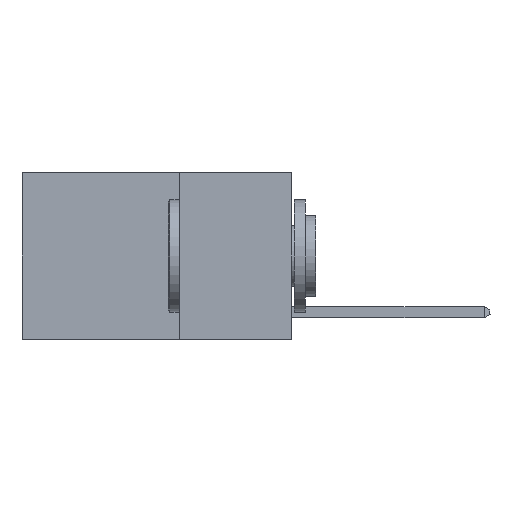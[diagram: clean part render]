
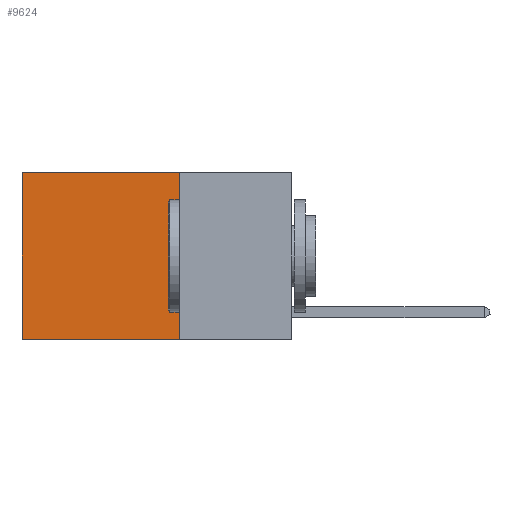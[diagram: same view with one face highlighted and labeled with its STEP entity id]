
A CAD part, left-side view. The second image highlights one B-rep face of the part: STEP entity #9624.
In plain terms, the highlighted planar face has unit normal (-1, 0, 0).
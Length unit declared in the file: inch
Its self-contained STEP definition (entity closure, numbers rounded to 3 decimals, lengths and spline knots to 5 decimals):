
#77 = AXIS2_PLACEMENT_3D ( 'NONE', #5192, #1181, #6206 ) ;
#210 = ORIENTED_EDGE ( 'NONE', *, *, #11978, .F. ) ;
#230 = CARTESIAN_POINT ( 'NONE',  ( 0.2625, 0.6, 0. ) ) ;
#851 = CARTESIAN_POINT ( 'NONE',  ( 0.2625, 0.25, 0. ) ) ;
#937 = DIRECTION ( 'NONE',  ( 0., 0., -1. ) ) ;
#1181 = DIRECTION ( 'NONE',  ( 1., 0., 0. ) ) ;
#1948 = CARTESIAN_POINT ( 'NONE',  ( 0.2625, 0.25, -0.37 ) ) ;
#1982 = VECTOR ( 'NONE', #937, 39.37008 ) ;
#2032 = VERTEX_POINT ( 'NONE', #7979 ) ;
#2310 = VECTOR ( 'NONE', #5855, 39.37008 ) ;
#2860 = DIRECTION ( 'NONE',  ( 0., 1., 0. ) ) ;
#2877 = LINE ( 'NONE', #1948, #3888 ) ;
#2920 = ORIENTED_EDGE ( 'NONE', *, *, #11992, .F. ) ;
#3165 = CARTESIAN_POINT ( 'NONE',  ( 0.2625, 0.25, -0.37 ) ) ;
#3554 = ORIENTED_EDGE ( 'NONE', *, *, #11331, .T. ) ;
#3816 = DIRECTION ( 'NONE',  ( 0., 1., 0. ) ) ;
#3888 = VECTOR ( 'NONE', #3816, 39.37008 ) ;
#4847 = CARTESIAN_POINT ( 'NONE',  ( 0.2625, 0.6, 0. ) ) ;
#4977 = LINE ( 'NONE', #4847, #2310 ) ;
#5192 = CARTESIAN_POINT ( 'NONE',  ( 0.2625, 0.25, 0. ) ) ;
#5855 = DIRECTION ( 'NONE',  ( 0., 0., -1. ) ) ;
#6206 = DIRECTION ( 'NONE',  ( 0., 0., -1. ) ) ;
#6702 = VERTEX_POINT ( 'NONE', #3165 ) ;
#6823 = LINE ( 'NONE', #7877, #1982 ) ;
#6914 = EDGE_CURVE ( 'NONE', #7599, #2032, #4977, .T. ) ;
#7201 = FACE_OUTER_BOUND ( 'NONE', #10203, .T. ) ;
#7398 = CARTESIAN_POINT ( 'NONE',  ( 0.2625, 0.25, 0. ) ) ;
#7599 = VERTEX_POINT ( 'NONE', #230 ) ;
#7877 = CARTESIAN_POINT ( 'NONE',  ( 0.2625, 0.25, 0. ) ) ;
#7979 = CARTESIAN_POINT ( 'NONE',  ( 0.2625, 0.6, -0.37 ) ) ;
#8109 = VERTEX_POINT ( 'NONE', #7398 ) ;
#8574 = ORIENTED_EDGE ( 'NONE', *, *, #6914, .T. ) ;
#9062 = PLANE ( 'NONE',  #77 ) ;
#9195 = VECTOR ( 'NONE', #2860, 39.37008 ) ;
#9624 = ADVANCED_FACE ( 'NONE', ( #7201 ), #9062, .F. ) ;
#9915 = LINE ( 'NONE', #851, #9195 ) ;
#10203 = EDGE_LOOP ( 'NONE', ( #8574, #210, #2920, #3554 ) ) ;
#11331 = EDGE_CURVE ( 'NONE', #8109, #7599, #9915, .T. ) ;
#11978 = EDGE_CURVE ( 'NONE', #6702, #2032, #2877, .T. ) ;
#11992 = EDGE_CURVE ( 'NONE', #8109, #6702, #6823, .T. ) ;
